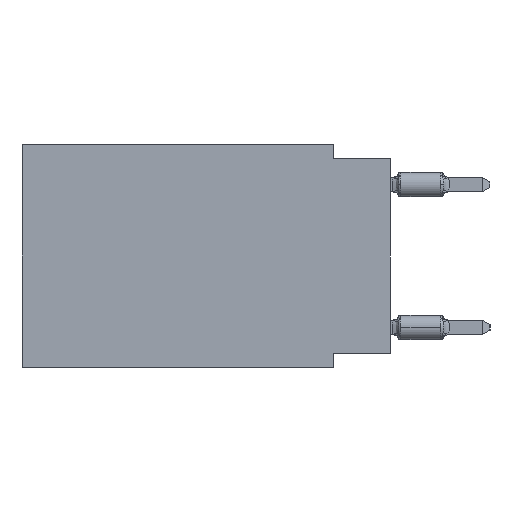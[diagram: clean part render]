
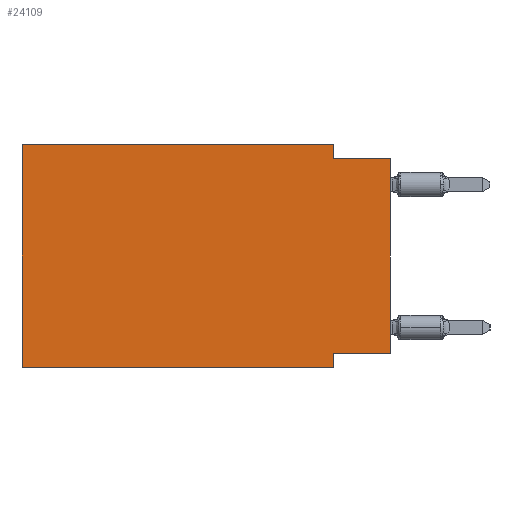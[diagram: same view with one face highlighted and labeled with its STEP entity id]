
A CAD part, left-side view. The second image highlights one B-rep face of the part: STEP entity #24109.
In plain terms, the highlighted planar face has unit normal (-1, 0, 0).
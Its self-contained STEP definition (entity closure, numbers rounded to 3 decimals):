
#372 = DIRECTION ( 'NONE',  ( 0., 0., 1. ) ) ;
#852 = DIRECTION ( 'NONE',  ( 0., 0., -1. ) ) ;
#1183 = EDGE_CURVE ( 'NONE', #27431, #3493, #30016, .T. ) ;
#1617 = VECTOR ( 'NONE', #10061, 1000. ) ;
#2798 = LINE ( 'NONE', #21143, #33351 ) ;
#2801 = VERTEX_POINT ( 'NONE', #8240 ) ;
#3449 = LINE ( 'NONE', #21808, #15872 ) ;
#3493 = VERTEX_POINT ( 'NONE', #13234 ) ;
#3781 = ORIENTED_EDGE ( 'NONE', *, *, #25710, .F. ) ;
#4200 = AXIS2_PLACEMENT_3D ( 'NONE', #8642, #32673, #852 ) ;
#5086 = EDGE_CURVE ( 'NONE', #3493, #2801, #18245, .T. ) ;
#5991 = DIRECTION ( 'NONE',  ( 0., -1., 0. ) ) ;
#6575 = ORIENTED_EDGE ( 'NONE', *, *, #1183, .F. ) ;
#6628 = CARTESIAN_POINT ( 'NONE',  ( 0., 16.383, -9.906 ) ) ;
#8240 = CARTESIAN_POINT ( 'NONE',  ( 0., 2.54, -9.906 ) ) ;
#8642 = CARTESIAN_POINT ( 'NONE',  ( 0., 16.383, 0. ) ) ;
#9171 = CARTESIAN_POINT ( 'NONE',  ( 0., 2.54, -9.906 ) ) ;
#9710 = EDGE_CURVE ( 'NONE', #18755, #23232, #29582, .T. ) ;
#9959 = VERTEX_POINT ( 'NONE', #12770 ) ;
#10061 = DIRECTION ( 'NONE',  ( 0., -1., 0. ) ) ;
#10377 = DIRECTION ( 'NONE',  ( 0., 0., 1. ) ) ;
#10918 = CARTESIAN_POINT ( 'NONE',  ( 0., 2.54, -0.635 ) ) ;
#11555 = EDGE_CURVE ( 'NONE', #27431, #34144, #23201, .T. ) ;
#11600 = DIRECTION ( 'NONE',  ( 0., 0., -1. ) ) ;
#12090 = VECTOR ( 'NONE', #27430, 1000. ) ;
#12770 = CARTESIAN_POINT ( 'NONE',  ( 0., 2.54, 0. ) ) ;
#13234 = CARTESIAN_POINT ( 'NONE',  ( 0., 2.54, -9.271 ) ) ;
#13591 = LINE ( 'NONE', #29679, #18406 ) ;
#14734 = EDGE_CURVE ( 'NONE', #23232, #9959, #13591, .T. ) ;
#15586 = ORIENTED_EDGE ( 'NONE', *, *, #11555, .T. ) ;
#15872 = VECTOR ( 'NONE', #11600, 1000. ) ;
#16289 = EDGE_LOOP ( 'NONE', ( #15586, #20451, #3781, #27542, #25264, #31240, #30080, #6575 ) ) ;
#16552 = CARTESIAN_POINT ( 'NONE',  ( 0., 0., -0.635 ) ) ;
#16865 = CARTESIAN_POINT ( 'NONE',  ( 0., 0., -9.271 ) ) ;
#17841 = CARTESIAN_POINT ( 'NONE',  ( 0., 16.383, -9.906 ) ) ;
#18245 = LINE ( 'NONE', #9171, #34119 ) ;
#18406 = VECTOR ( 'NONE', #5991, 1000. ) ;
#18755 = VERTEX_POINT ( 'NONE', #6628 ) ;
#18916 = CARTESIAN_POINT ( 'NONE',  ( 0., 16.383, 0. ) ) ;
#19124 = VECTOR ( 'NONE', #10377, 1000. ) ;
#20336 = EDGE_CURVE ( 'NONE', #18755, #2801, #33607, .T. ) ;
#20451 = ORIENTED_EDGE ( 'NONE', *, *, #31282, .F. ) ;
#21143 = CARTESIAN_POINT ( 'NONE',  ( 0., 0., -0.635 ) ) ;
#21808 = CARTESIAN_POINT ( 'NONE',  ( 0., 2.54, 0. ) ) ;
#22331 = VECTOR ( 'NONE', #372, 1000. ) ;
#23201 = LINE ( 'NONE', #34069, #19124 ) ;
#23232 = VERTEX_POINT ( 'NONE', #18916 ) ;
#23522 = CARTESIAN_POINT ( 'NONE',  ( 0., 0., -9.271 ) ) ;
#24058 = CARTESIAN_POINT ( 'NONE',  ( 0., 16.383, 0. ) ) ;
#24109 = ADVANCED_FACE ( 'NONE', ( #32858 ), #29559, .F. ) ;
#25264 = ORIENTED_EDGE ( 'NONE', *, *, #9710, .F. ) ;
#25710 = EDGE_CURVE ( 'NONE', #9959, #32418, #3449, .T. ) ;
#27430 = DIRECTION ( 'NONE',  ( 0., 1., 0. ) ) ;
#27431 = VERTEX_POINT ( 'NONE', #23522 ) ;
#27542 = ORIENTED_EDGE ( 'NONE', *, *, #14734, .F. ) ;
#29559 = PLANE ( 'NONE',  #4200 ) ;
#29582 = LINE ( 'NONE', #24058, #22331 ) ;
#29679 = CARTESIAN_POINT ( 'NONE',  ( 0., 16.383, 0. ) ) ;
#30016 = LINE ( 'NONE', #16865, #12090 ) ;
#30080 = ORIENTED_EDGE ( 'NONE', *, *, #5086, .F. ) ;
#31240 = ORIENTED_EDGE ( 'NONE', *, *, #20336, .T. ) ;
#31282 = EDGE_CURVE ( 'NONE', #32418, #34144, #2798, .T. ) ;
#31682 = DIRECTION ( 'NONE',  ( 0., -1., 0. ) ) ;
#32418 = VERTEX_POINT ( 'NONE', #10918 ) ;
#32673 = DIRECTION ( 'NONE',  ( 1., 0., 0. ) ) ;
#32858 = FACE_OUTER_BOUND ( 'NONE', #16289, .T. ) ;
#33351 = VECTOR ( 'NONE', #31682, 1000. ) ;
#33607 = LINE ( 'NONE', #17841, #1617 ) ;
#33831 = DIRECTION ( 'NONE',  ( 0., 0., -1. ) ) ;
#34069 = CARTESIAN_POINT ( 'NONE',  ( 0., 0., 0. ) ) ;
#34119 = VECTOR ( 'NONE', #33831, 1000. ) ;
#34144 = VERTEX_POINT ( 'NONE', #16552 ) ;
